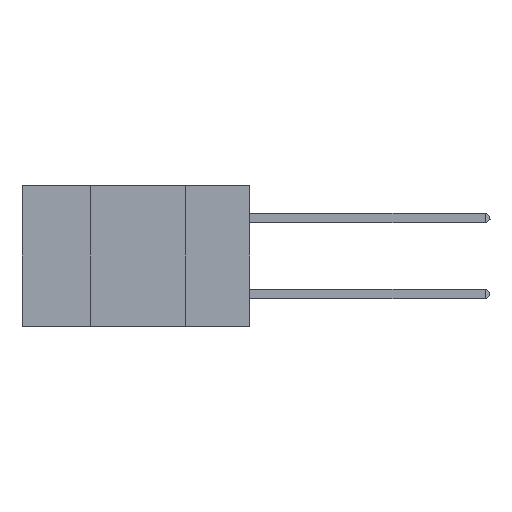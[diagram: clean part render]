
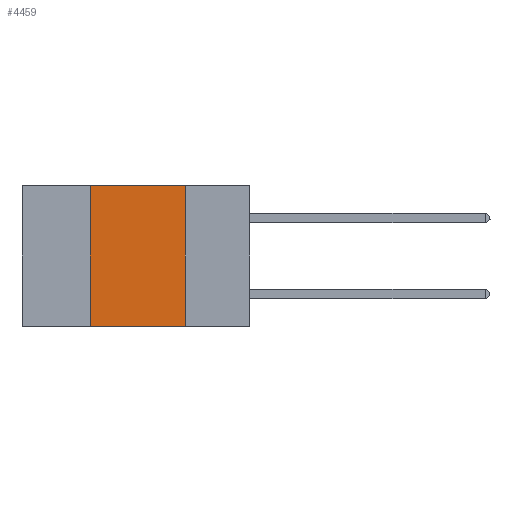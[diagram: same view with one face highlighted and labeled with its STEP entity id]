
A CAD part, left-side view. The second image highlights one B-rep face of the part: STEP entity #4459.
In plain terms, the highlighted planar face has unit normal (-1, 0, 0).
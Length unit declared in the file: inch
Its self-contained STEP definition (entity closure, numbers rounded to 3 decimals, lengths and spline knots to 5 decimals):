
#640 = EDGE_LOOP ( 'NONE', ( #24846, #5389, #10634, #26178 ) ) ;
#1194 = LINE ( 'NONE', #12993, #20243 ) ;
#1357 = DIRECTION ( 'NONE',  ( 0., -1., 0. ) ) ;
#1366 = PLANE ( 'NONE',  #6887 ) ;
#1945 = EDGE_CURVE ( 'NONE', #24841, #13526, #30593, .T. ) ;
#2601 = EDGE_CURVE ( 'NONE', #24841, #24157, #22847, .T. ) ;
#3072 = CARTESIAN_POINT ( 'NONE',  ( 0., 0.42, -0.37 ) ) ;
#3385 = CARTESIAN_POINT ( 'NONE',  ( 0., 0.42, 0. ) ) ;
#4459 = ADVANCED_FACE ( 'NONE', ( #12257 ), #1366, .F. ) ;
#5389 = ORIENTED_EDGE ( 'NONE', *, *, #31880, .F. ) ;
#6887 = AXIS2_PLACEMENT_3D ( 'NONE', #28808, #15977, #8912 ) ;
#7970 = DIRECTION ( 'NONE',  ( 0., 0., 1. ) ) ;
#8912 = DIRECTION ( 'NONE',  ( 0., 0., -1. ) ) ;
#9788 = VECTOR ( 'NONE', #1357, 39.37008 ) ;
#10634 = ORIENTED_EDGE ( 'NONE', *, *, #2601, .F. ) ;
#11302 = VERTEX_POINT ( 'NONE', #15062 ) ;
#12257 = FACE_OUTER_BOUND ( 'NONE', #640, .T. ) ;
#12993 = CARTESIAN_POINT ( 'NONE',  ( 0., 0.17, 0. ) ) ;
#13526 = VERTEX_POINT ( 'NONE', #21156 ) ;
#13665 = CARTESIAN_POINT ( 'NONE',  ( 0., 0.42, 0. ) ) ;
#15062 = CARTESIAN_POINT ( 'NONE',  ( 0., 0.17, 0. ) ) ;
#15626 = DIRECTION ( 'NONE',  ( 0., 0., -1. ) ) ;
#15977 = DIRECTION ( 'NONE',  ( 1., 0., 0. ) ) ;
#19469 = CARTESIAN_POINT ( 'NONE',  ( 0., 0.6, 0. ) ) ;
#20243 = VECTOR ( 'NONE', #15626, 39.37008 ) ;
#21156 = CARTESIAN_POINT ( 'NONE',  ( 0., 0.17, -0.37 ) ) ;
#22847 = LINE ( 'NONE', #3385, #26520 ) ;
#24157 = VERTEX_POINT ( 'NONE', #13665 ) ;
#24341 = DIRECTION ( 'NONE',  ( 0., -1., 0. ) ) ;
#24841 = VERTEX_POINT ( 'NONE', #3072 ) ;
#24846 = ORIENTED_EDGE ( 'NONE', *, *, #29587, .F. ) ;
#26178 = ORIENTED_EDGE ( 'NONE', *, *, #1945, .T. ) ;
#26203 = CARTESIAN_POINT ( 'NONE',  ( 0., 0.6, -0.37 ) ) ;
#26520 = VECTOR ( 'NONE', #7970, 39.37008 ) ;
#28808 = CARTESIAN_POINT ( 'NONE',  ( 0., 0.6, 0. ) ) ;
#29047 = LINE ( 'NONE', #19469, #32192 ) ;
#29587 = EDGE_CURVE ( 'NONE', #11302, #13526, #1194, .T. ) ;
#30593 = LINE ( 'NONE', #26203, #9788 ) ;
#31880 = EDGE_CURVE ( 'NONE', #24157, #11302, #29047, .T. ) ;
#32192 = VECTOR ( 'NONE', #24341, 39.37008 ) ;
